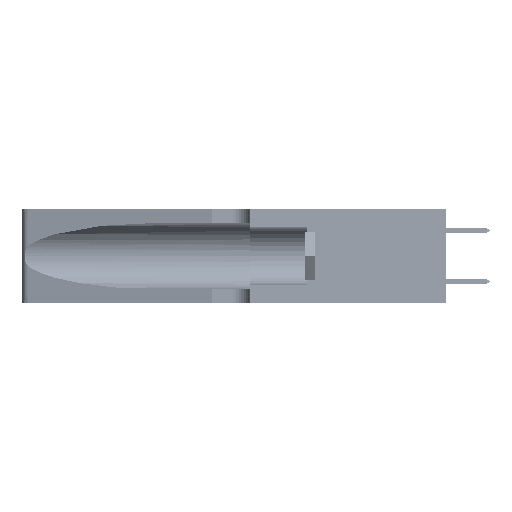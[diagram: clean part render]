
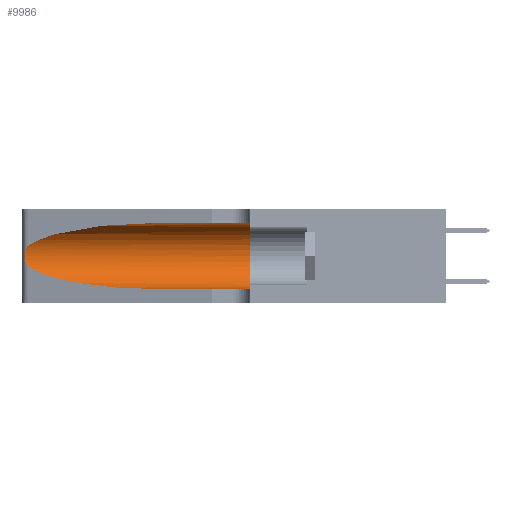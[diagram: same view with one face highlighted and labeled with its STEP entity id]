
A CAD part, left-side view. The second image highlights one B-rep face of the part: STEP entity #9986.
In plain terms, the highlighted cylindrical face has radius 3.308 mm (diameter 6.617 mm), a partial arc.
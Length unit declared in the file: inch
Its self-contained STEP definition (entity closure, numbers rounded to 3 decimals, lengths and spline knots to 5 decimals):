
#1016 = FACE_OUTER_BOUND ( 'NONE', #32404, .T. ) ;
#1207 = EDGE_CURVE ( 'NONE', #13879, #14230, #18527, .T. ) ;
#1292 = CARTESIAN_POINT ( 'NONE',  ( 0.1305, 0.72297, 0.31525 ) ) ;
#3232 = CARTESIAN_POINT ( 'NONE',  ( 0.26017, 1.23833, 0.17102 ) ) ;
#3465 = DIRECTION ( 'NONE',  ( 0., -1., 0. ) ) ;
#3637 = VECTOR ( 'NONE', #17206, 39.37008 ) ;
#3792 = ORIENTED_EDGE ( 'NONE', *, *, #26091, .F. ) ;
#4544 = DIRECTION ( 'NONE',  ( 0., 1., 0. ) ) ;
#4948 = LINE ( 'NONE', #13015, #3637 ) ;
#5331 = EDGE_CURVE ( 'NONE', #14230, #37916, #4948, .T. ) ;
#7208 = CARTESIAN_POINT ( 'NONE',  ( 0.25487, 1.22718, 0.22369 ) ) ;
#7390 = CARTESIAN_POINT ( 'NONE',  ( 0.25789, 1.23486, 0.15765 ) ) ;
#8411 = LINE ( 'NONE', #25037, #20890 ) ;
#9986 = ADVANCED_FACE ( 'NONE', ( #1016 ), #33233, .F. ) ;
#9994 = CARTESIAN_POINT ( 'NONE',  ( 0.2373, 1.15595, 0.08982 ) ) ;
#11279 = ORIENTED_EDGE ( 'NONE', *, *, #27864, .T. ) ;
#11437 = CARTESIAN_POINT ( 'NONE',  ( 0.25555, 1.22994, 0.2215 ) ) ;
#11616 = CARTESIAN_POINT ( 'NONE',  ( 0.25555, 1.22993, 0.14849 ) ) ;
#13015 = CARTESIAN_POINT ( 'NONE',  ( 0.1305, 1.61858, 0.05475 ) ) ;
#13879 = VERTEX_POINT ( 'NONE', #51399 ) ;
#14230 = VERTEX_POINT ( 'NONE', #25252 ) ;
#14236 = CARTESIAN_POINT ( 'NONE',  ( 0.1305, 0.72297, 0.05475 ) ) ;
#14495 = B_SPLINE_CURVE_WITH_KNOTS ( 'NONE', 3,
 ( #7208, #11437, #44979, #19876, #49183, #24143, #53384, #28381, #3232, #32617, #7390, #36798, #11616, #40974 ),
 .UNSPECIFIED., .F., .F.,
 ( 4, 2, 2, 2, 2, 2, 4 ),
 ( 0., 0.00027, 0.00053, 0.00107, 0.0016, 0.00187, 0.00214 ),
 .UNSPECIFIED. ) ;
#17206 = DIRECTION ( 'NONE',  ( 0., -1., 0. ) ) ;
#18527 =( BOUNDED_CURVE ( )  B_SPLINE_CURVE ( 3, ( #39376, #9994, #31010, #14236 ),
 .UNSPECIFIED., .F., .F. ) 
 B_SPLINE_CURVE_WITH_KNOTS ( ( 4, 4 ),
 ( 3.44316, 4.71239 ),
 .UNSPECIFIED. ) 
 CURVE ( )  GEOMETRIC_REPRESENTATION_ITEM ( )  RATIONAL_B_SPLINE_CURVE ( ( 1., 0.87, 0.87, 1. ) ) 
 REPRESENTATION_ITEM ( '' )  );
#19876 = CARTESIAN_POINT ( 'NONE',  ( 0.25787, 1.23484, 0.2124 ) ) ;
#20126 = CARTESIAN_POINT ( 'NONE',  ( 0.1305, 1.61858, 0.185 ) ) ;
#20890 = VECTOR ( 'NONE', #41671, 39.37008 ) ;
#21077 = AXIS2_PLACEMENT_3D ( 'NONE', #20126, #3465, #32849 ) ;
#22313 = EDGE_CURVE ( 'NONE', #40330, #37916, #25686, .T. ) ;
#22356 = CARTESIAN_POINT ( 'NONE',  ( 0.2373, 1.15595, 0.28018 ) ) ;
#22563 = AXIS2_PLACEMENT_3D ( 'NONE', #29731, #4544, #33942 ) ;
#24143 = CARTESIAN_POINT ( 'NONE',  ( 0.26018, 1.23835, 0.19895 ) ) ;
#25037 = CARTESIAN_POINT ( 'NONE',  ( 0.1305, 1.61858, 0.31525 ) ) ;
#25252 = CARTESIAN_POINT ( 'NONE',  ( 0.1305, 0.72297, 0.05475 ) ) ;
#25532 = ORIENTED_EDGE ( 'NONE', *, *, #5331, .T. ) ;
#25686 = CIRCLE ( 'NONE', #22563, 0.13025 ) ;
#26091 = EDGE_CURVE ( 'NONE', #44512, #40330, #8411, .T. ) ;
#26170 = CARTESIAN_POINT ( 'NONE',  ( 0.1305, 0.35, 0.31525 ) ) ;
#26445 = CARTESIAN_POINT ( 'NONE',  ( 0.18966, 0.96281, 0.31525 ) ) ;
#27178 = VERTEX_POINT ( 'NONE', #35951 ) ;
#27864 = EDGE_CURVE ( 'NONE', #27178, #13879, #14495, .T. ) ;
#28381 = CARTESIAN_POINT ( 'NONE',  ( 0.26075, 1.23896, 0.178 ) ) ;
#29731 = CARTESIAN_POINT ( 'NONE',  ( 0.1305, 0.35, 0.185 ) ) ;
#31010 = CARTESIAN_POINT ( 'NONE',  ( 0.18966, 0.96281, 0.05475 ) ) ;
#31739 = ORIENTED_EDGE ( 'NONE', *, *, #1207, .T. ) ;
#32404 = EDGE_LOOP ( 'NONE', ( #37824, #11279, #31739, #25532, #39985, #3792 ) ) ;
#32617 = CARTESIAN_POINT ( 'NONE',  ( 0.25856, 1.23593, 0.16098 ) ) ;
#32849 = DIRECTION ( 'NONE',  ( 0., 0., -1. ) ) ;
#33233 = CYLINDRICAL_SURFACE ( 'NONE', #21077, 0.13025 ) ;
#33942 = DIRECTION ( 'NONE',  ( 0., 0., 1. ) ) ;
#35753 =( BOUNDED_CURVE ( )  B_SPLINE_CURVE ( 3, ( #1292, #26445, #22356, #51643 ),
 .UNSPECIFIED., .F., .F. ) 
 B_SPLINE_CURVE_WITH_KNOTS ( ( 4, 4 ),
 ( 1.5708, 2.84003 ),
 .UNSPECIFIED. ) 
 CURVE ( )  GEOMETRIC_REPRESENTATION_ITEM ( )  RATIONAL_B_SPLINE_CURVE ( ( 1., 0.87, 0.87, 1. ) ) 
 REPRESENTATION_ITEM ( '' )  );
#35951 = CARTESIAN_POINT ( 'NONE',  ( 0.25487, 1.22718, 0.22369 ) ) ;
#36798 = CARTESIAN_POINT ( 'NONE',  ( 0.25639, 1.23186, 0.15144 ) ) ;
#37824 = ORIENTED_EDGE ( 'NONE', *, *, #50887, .T. ) ;
#37916 = VERTEX_POINT ( 'NONE', #46996 ) ;
#39376 = CARTESIAN_POINT ( 'NONE',  ( 0.25487, 1.22718, 0.14631 ) ) ;
#39985 = ORIENTED_EDGE ( 'NONE', *, *, #22313, .F. ) ;
#40330 = VERTEX_POINT ( 'NONE', #26170 ) ;
#40839 = CARTESIAN_POINT ( 'NONE',  ( 0.1305, 0.72297, 0.31525 ) ) ;
#40974 = CARTESIAN_POINT ( 'NONE',  ( 0.25487, 1.22718, 0.14631 ) ) ;
#41671 = DIRECTION ( 'NONE',  ( 0., -1., 0. ) ) ;
#44512 = VERTEX_POINT ( 'NONE', #40839 ) ;
#44979 = CARTESIAN_POINT ( 'NONE',  ( 0.25639, 1.23184, 0.21858 ) ) ;
#46996 = CARTESIAN_POINT ( 'NONE',  ( 0.1305, 0.35, 0.05475 ) ) ;
#49183 = CARTESIAN_POINT ( 'NONE',  ( 0.25854, 1.2359, 0.20912 ) ) ;
#50887 = EDGE_CURVE ( 'NONE', #44512, #27178, #35753, .T. ) ;
#51399 = CARTESIAN_POINT ( 'NONE',  ( 0.25487, 1.22718, 0.14631 ) ) ;
#51643 = CARTESIAN_POINT ( 'NONE',  ( 0.25487, 1.22718, 0.22369 ) ) ;
#53384 = CARTESIAN_POINT ( 'NONE',  ( 0.26075, 1.23896, 0.19203 ) ) ;
